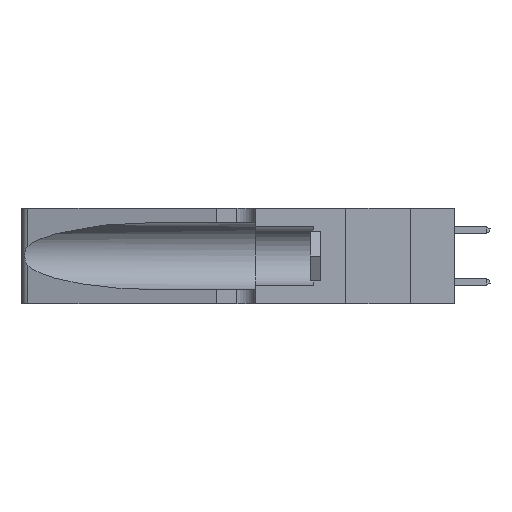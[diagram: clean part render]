
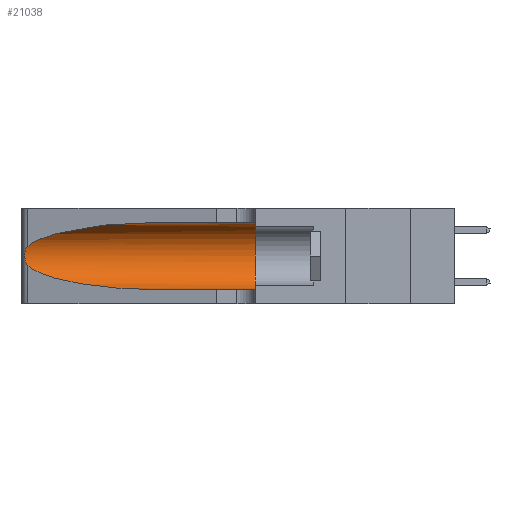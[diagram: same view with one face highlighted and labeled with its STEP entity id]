
A CAD part, left-side view. The second image highlights one B-rep face of the part: STEP entity #21038.
In plain terms, the highlighted cylindrical face has radius 3.308 mm (diameter 6.617 mm), a partial arc.
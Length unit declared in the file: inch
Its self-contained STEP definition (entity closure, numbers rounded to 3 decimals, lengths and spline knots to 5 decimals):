
#256 = VECTOR ( 'NONE', #23867, 39.37008 ) ;
#270 = CARTESIAN_POINT ( 'NONE',  ( 0.18966, 0.96281, 0.05475 ) ) ;
#1144 = CARTESIAN_POINT ( 'NONE',  ( 0.1305, 0.72297, 0.31525 ) ) ;
#1165 = CARTESIAN_POINT ( 'NONE',  ( 0.25487, 1.22718, 0.14631 ) ) ;
#1448 = VERTEX_POINT ( 'NONE', #11612 ) ;
#1520 = CARTESIAN_POINT ( 'NONE',  ( 0.1305, 1.61858, 0.05475 ) ) ;
#2262 = CARTESIAN_POINT ( 'NONE',  ( 0.25639, 1.23184, 0.21858 ) ) ;
#2731 = EDGE_CURVE ( 'NONE', #1448, #33779, #36107, .T. ) ;
#2952 = ORIENTED_EDGE ( 'NONE', *, *, #6442, .F. ) ;
#3309 = EDGE_LOOP ( 'NONE', ( #32425, #21463, #36383, #33446, #12099, #2952 ) ) ;
#5671 = CARTESIAN_POINT ( 'NONE',  ( 0.25856, 1.23593, 0.16098 ) ) ;
#6000 = CARTESIAN_POINT ( 'NONE',  ( 0.2373, 1.15595, 0.08982 ) ) ;
#6442 = EDGE_CURVE ( 'NONE', #7813, #27953, #28705, .T. ) ;
#6693 = FACE_OUTER_BOUND ( 'NONE', #3309, .T. ) ;
#7447 = CARTESIAN_POINT ( 'NONE',  ( 0.1305, 1.61858, 0.185 ) ) ;
#7591 = DIRECTION ( 'NONE',  ( 0., 0., 1. ) ) ;
#7702 = DIRECTION ( 'NONE',  ( 0., 0., -1. ) ) ;
#7813 = VERTEX_POINT ( 'NONE', #1144 ) ;
#8200 = CARTESIAN_POINT ( 'NONE',  ( 0.26075, 1.23896, 0.178 ) ) ;
#8323 = VERTEX_POINT ( 'NONE', #31110 ) ;
#8763 = CARTESIAN_POINT ( 'NONE',  ( 0.25487, 1.22718, 0.14631 ) ) ;
#8790 =( BOUNDED_CURVE ( )  B_SPLINE_CURVE ( 3, ( #26231, #14766, #32453, #17794 ),
 .UNSPECIFIED., .F., .T. ) 
 B_SPLINE_CURVE_WITH_KNOTS ( ( 4, 4 ),
 ( 1.5708, 2.84003 ),
 .UNSPECIFIED. ) 
 CURVE ( )  GEOMETRIC_REPRESENTATION_ITEM ( )  RATIONAL_B_SPLINE_CURVE ( ( 1., 0.87, 0.87, 1. ) ) 
 REPRESENTATION_ITEM ( '' )  );
#9389 = CARTESIAN_POINT ( 'NONE',  ( 0.1305, 1.61858, 0.31525 ) ) ;
#10276 = VERTEX_POINT ( 'NONE', #1165 ) ;
#11612 = CARTESIAN_POINT ( 'NONE',  ( 0.1305, 0.72297, 0.05475 ) ) ;
#11629 = CYLINDRICAL_SURFACE ( 'NONE', #35516, 0.13025 ) ;
#12099 = ORIENTED_EDGE ( 'NONE', *, *, #30461, .F. ) ;
#12786 = CIRCLE ( 'NONE', #35106, 0.13025 ) ;
#13086 = CARTESIAN_POINT ( 'NONE',  ( 0.1305, 0.35, 0.185 ) ) ;
#14766 = CARTESIAN_POINT ( 'NONE',  ( 0.18966, 0.96281, 0.31525 ) ) ;
#15866 = DIRECTION ( 'NONE',  ( 0., -1., 0. ) ) ;
#16962 = CARTESIAN_POINT ( 'NONE',  ( 0.26018, 1.23835, 0.19895 ) ) ;
#17459 = CARTESIAN_POINT ( 'NONE',  ( 0.25555, 1.22993, 0.14849 ) ) ;
#17552 = EDGE_CURVE ( 'NONE', #7813, #8323, #8790, .T. ) ;
#17794 = CARTESIAN_POINT ( 'NONE',  ( 0.25487, 1.22718, 0.22369 ) ) ;
#19296 = DIRECTION ( 'NONE',  ( 0., 1., 0. ) ) ;
#20566 = B_SPLINE_CURVE_WITH_KNOTS ( 'NONE', 3,
 ( #28060, #36960, #2262, #31039, #34171, #16962, #36822, #8200, #22932, #5671, #31397, #22805, #17459, #34669 ),
 .UNSPECIFIED., .F., .F.,
 ( 4, 2, 2, 2, 2, 2, 4 ),
 ( 0., 0.00027, 0.00053, 0.00107, 0.0016, 0.00187, 0.00214 ),
 .UNSPECIFIED. ) ;
#20710 = CARTESIAN_POINT ( 'NONE',  ( 0.1305, 0.35, 0.31525 ) ) ;
#21038 = ADVANCED_FACE ( 'NONE', ( #6693 ), #11629, .F. ) ;
#21251 = EDGE_CURVE ( 'NONE', #8323, #10276, #20566, .T. ) ;
#21463 = ORIENTED_EDGE ( 'NONE', *, *, #21251, .T. ) ;
#22031 = EDGE_CURVE ( 'NONE', #10276, #1448, #29972, .T. ) ;
#22805 = CARTESIAN_POINT ( 'NONE',  ( 0.25639, 1.23186, 0.15144 ) ) ;
#22932 = CARTESIAN_POINT ( 'NONE',  ( 0.26017, 1.23833, 0.17102 ) ) ;
#23867 = DIRECTION ( 'NONE',  ( 0., -1., 0. ) ) ;
#26231 = CARTESIAN_POINT ( 'NONE',  ( 0.1305, 0.72297, 0.31525 ) ) ;
#26346 = CARTESIAN_POINT ( 'NONE',  ( 0.1305, 0.72297, 0.05475 ) ) ;
#27029 = CARTESIAN_POINT ( 'NONE',  ( 0.1305, 0.35, 0.05475 ) ) ;
#27334 = DIRECTION ( 'NONE',  ( 0., -1., 0. ) ) ;
#27953 = VERTEX_POINT ( 'NONE', #20710 ) ;
#28060 = CARTESIAN_POINT ( 'NONE',  ( 0.25487, 1.22718, 0.22369 ) ) ;
#28499 = VECTOR ( 'NONE', #27334, 39.37008 ) ;
#28705 = LINE ( 'NONE', #9389, #256 ) ;
#29972 =( BOUNDED_CURVE ( )  B_SPLINE_CURVE ( 3, ( #8763, #6000, #270, #26346 ),
 .UNSPECIFIED., .F., .F. ) 
 B_SPLINE_CURVE_WITH_KNOTS ( ( 4, 4 ),
 ( 3.44316, 4.71239 ),
 .UNSPECIFIED. ) 
 CURVE ( )  GEOMETRIC_REPRESENTATION_ITEM ( )  RATIONAL_B_SPLINE_CURVE ( ( 1., 0.87, 0.87, 1. ) ) 
 REPRESENTATION_ITEM ( '' )  );
#30461 = EDGE_CURVE ( 'NONE', #27953, #33779, #12786, .T. ) ;
#31039 = CARTESIAN_POINT ( 'NONE',  ( 0.25787, 1.23484, 0.2124 ) ) ;
#31110 = CARTESIAN_POINT ( 'NONE',  ( 0.25487, 1.22718, 0.22369 ) ) ;
#31397 = CARTESIAN_POINT ( 'NONE',  ( 0.25789, 1.23486, 0.15765 ) ) ;
#32425 = ORIENTED_EDGE ( 'NONE', *, *, #17552, .T. ) ;
#32453 = CARTESIAN_POINT ( 'NONE',  ( 0.2373, 1.15595, 0.28018 ) ) ;
#33446 = ORIENTED_EDGE ( 'NONE', *, *, #2731, .T. ) ;
#33779 = VERTEX_POINT ( 'NONE', #27029 ) ;
#34171 = CARTESIAN_POINT ( 'NONE',  ( 0.25854, 1.2359, 0.20912 ) ) ;
#34669 = CARTESIAN_POINT ( 'NONE',  ( 0.25487, 1.22718, 0.14631 ) ) ;
#35106 = AXIS2_PLACEMENT_3D ( 'NONE', #13086, #19296, #7591 ) ;
#35516 = AXIS2_PLACEMENT_3D ( 'NONE', #7447, #15866, #7702 ) ;
#36107 = LINE ( 'NONE', #1520, #28499 ) ;
#36383 = ORIENTED_EDGE ( 'NONE', *, *, #22031, .T. ) ;
#36822 = CARTESIAN_POINT ( 'NONE',  ( 0.26075, 1.23896, 0.19203 ) ) ;
#36960 = CARTESIAN_POINT ( 'NONE',  ( 0.25555, 1.22994, 0.2215 ) ) ;
